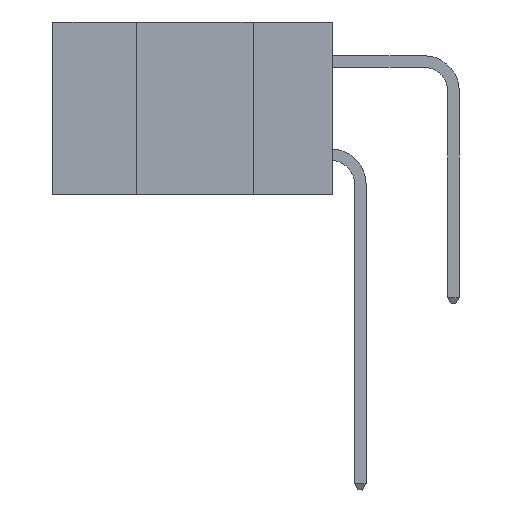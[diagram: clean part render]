
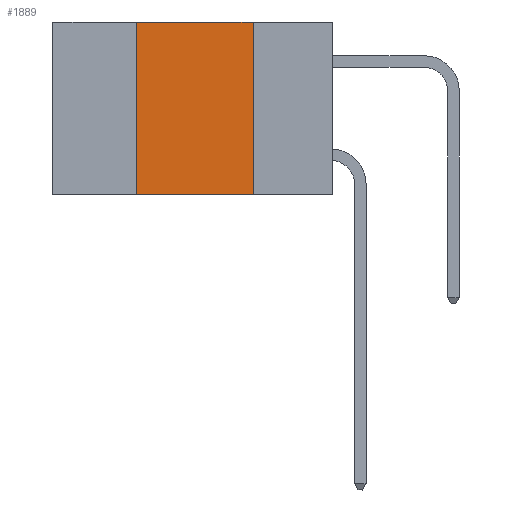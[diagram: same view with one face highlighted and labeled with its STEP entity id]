
A CAD part, left-side view. The second image highlights one B-rep face of the part: STEP entity #1889.
In plain terms, the highlighted planar face has unit normal (-1, 0, 0).
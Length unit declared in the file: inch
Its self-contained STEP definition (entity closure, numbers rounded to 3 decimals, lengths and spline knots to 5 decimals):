
#934 = VECTOR ( 'NONE', #9793, 39.37008 ) ;
#946 = FACE_OUTER_BOUND ( 'NONE', #1699, .T. ) ;
#1574 = DIRECTION ( 'NONE',  ( 0., 0., -1. ) ) ;
#1611 = CARTESIAN_POINT ( 'NONE',  ( 0., 0.17, 0. ) ) ;
#1699 = EDGE_LOOP ( 'NONE', ( #3571, #3614, #3778, #3841 ) ) ;
#1889 = ADVANCED_FACE ( 'NONE', ( #946 ), #17848, .F. ) ;
#2413 = EDGE_CURVE ( 'NONE', #5642, #12007, #4055, .T. ) ;
#2986 = LINE ( 'NONE', #1611, #10883 ) ;
#3571 = ORIENTED_EDGE ( 'NONE', *, *, #9408, .F. ) ;
#3614 = ORIENTED_EDGE ( 'NONE', *, *, #15990, .F. ) ;
#3778 = ORIENTED_EDGE ( 'NONE', *, *, #7371, .F. ) ;
#3841 = ORIENTED_EDGE ( 'NONE', *, *, #2413, .T. ) ;
#4055 = LINE ( 'NONE', #17040, #4987 ) ;
#4154 = CARTESIAN_POINT ( 'NONE',  ( 0., 0.42, -0.37 ) ) ;
#4476 = DIRECTION ( 'NONE',  ( 1., 0., 0. ) ) ;
#4481 = CARTESIAN_POINT ( 'NONE',  ( 0., 0.6, 0. ) ) ;
#4987 = VECTOR ( 'NONE', #17140, 39.37008 ) ;
#5442 = CARTESIAN_POINT ( 'NONE',  ( 0., 0.42, 0. ) ) ;
#5642 = VERTEX_POINT ( 'NONE', #4154 ) ;
#5813 = CARTESIAN_POINT ( 'NONE',  ( 0., 0.17, 0. ) ) ;
#7371 = EDGE_CURVE ( 'NONE', #5642, #12672, #10732, .T. ) ;
#9408 = EDGE_CURVE ( 'NONE', #17369, #12007, #2986, .T. ) ;
#9512 = DIRECTION ( 'NONE',  ( 0., 0., 1. ) ) ;
#9725 = CARTESIAN_POINT ( 'NONE',  ( 0., 0.42, 0. ) ) ;
#9793 = DIRECTION ( 'NONE',  ( 0., -1., 0. ) ) ;
#10732 = LINE ( 'NONE', #9725, #14626 ) ;
#10883 = VECTOR ( 'NONE', #1574, 39.37008 ) ;
#12007 = VERTEX_POINT ( 'NONE', #13316 ) ;
#12672 = VERTEX_POINT ( 'NONE', #5442 ) ;
#13316 = CARTESIAN_POINT ( 'NONE',  ( 0., 0.17, -0.37 ) ) ;
#14626 = VECTOR ( 'NONE', #9512, 39.37008 ) ;
#15516 = AXIS2_PLACEMENT_3D ( 'NONE', #4481, #4476, #18545 ) ;
#15670 = CARTESIAN_POINT ( 'NONE',  ( 0., 0.6, 0. ) ) ;
#15990 = EDGE_CURVE ( 'NONE', #12672, #17369, #17044, .T. ) ;
#17040 = CARTESIAN_POINT ( 'NONE',  ( 0., 0.6, -0.37 ) ) ;
#17044 = LINE ( 'NONE', #15670, #934 ) ;
#17140 = DIRECTION ( 'NONE',  ( 0., -1., 0. ) ) ;
#17369 = VERTEX_POINT ( 'NONE', #5813 ) ;
#17848 = PLANE ( 'NONE',  #15516 ) ;
#18545 = DIRECTION ( 'NONE',  ( 0., 0., -1. ) ) ;
